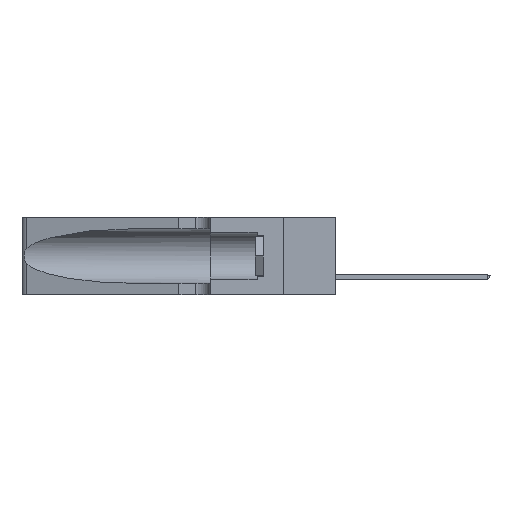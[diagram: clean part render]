
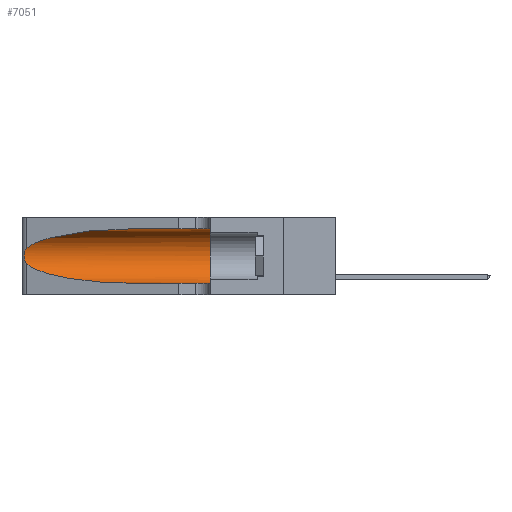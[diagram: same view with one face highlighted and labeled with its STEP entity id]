
A CAD part, left-side view. The second image highlights one B-rep face of the part: STEP entity #7051.
In plain terms, the highlighted cylindrical face has radius 3.308 mm (diameter 6.617 mm), a partial arc.
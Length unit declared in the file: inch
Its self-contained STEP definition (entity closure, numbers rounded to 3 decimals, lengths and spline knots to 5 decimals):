
#609 = CARTESIAN_POINT ( 'NONE',  ( 0.1305, 0.35, 0.31525 ) ) ;
#758 = CARTESIAN_POINT ( 'NONE',  ( 0.1305, 1.61858, 0.31525 ) ) ;
#1259 = AXIS2_PLACEMENT_3D ( 'NONE', #35674, #8339, #36142 ) ;
#1450 = CARTESIAN_POINT ( 'NONE',  ( 0.26075, 1.23896, 0.19203 ) ) ;
#2039 = CARTESIAN_POINT ( 'NONE',  ( 0.26075, 1.23896, 0.178 ) ) ;
#2385 = EDGE_CURVE ( 'NONE', #28341, #15840, #10176, .T. ) ;
#2926 = EDGE_CURVE ( 'NONE', #28791, #38067, #15833, .T. ) ;
#3540 = DIRECTION ( 'NONE',  ( 0., -1., 0. ) ) ;
#6143 = ORIENTED_EDGE ( 'NONE', *, *, #12284, .F. ) ;
#7031 = VERTEX_POINT ( 'NONE', #19176 ) ;
#7051 = ADVANCED_FACE ( 'NONE', ( #32981 ), #30847, .F. ) ;
#8081 = EDGE_CURVE ( 'NONE', #38067, #7031, #36028, .T. ) ;
#8339 = DIRECTION ( 'NONE',  ( 0., 1., 0. ) ) ;
#8526 = CARTESIAN_POINT ( 'NONE',  ( 0.26017, 1.23833, 0.17102 ) ) ;
#10176 = LINE ( 'NONE', #758, #22695 ) ;
#11030 = CARTESIAN_POINT ( 'NONE',  ( 0.1305, 0.72297, 0.31525 ) ) ;
#12284 = EDGE_CURVE ( 'NONE', #15840, #20941, #14368, .T. ) ;
#14368 = CIRCLE ( 'NONE', #1259, 0.13025 ) ;
#14975 = CARTESIAN_POINT ( 'NONE',  ( 0.25487, 1.22718, 0.22369 ) ) ;
#15460 = CARTESIAN_POINT ( 'NONE',  ( 0.25856, 1.23593, 0.16098 ) ) ;
#15833 = B_SPLINE_CURVE_WITH_KNOTS ( 'NONE', 3,
 ( #18590, #29553, #25940, #29239, #19055, #43270, #1450, #2039, #8526, #15460, #35856, #39640, #32686, #22611 ),
 .UNSPECIFIED., .F., .F.,
 ( 4, 2, 2, 2, 2, 2, 4 ),
 ( 0., 0.00027, 0.00053, 0.00107, 0.0016, 0.00187, 0.00214 ),
 .UNSPECIFIED. ) ;
#15840 = VERTEX_POINT ( 'NONE', #609 ) ;
#16563 = ORIENTED_EDGE ( 'NONE', *, *, #2926, .T. ) ;
#18590 = CARTESIAN_POINT ( 'NONE',  ( 0.25487, 1.22718, 0.22369 ) ) ;
#19055 = CARTESIAN_POINT ( 'NONE',  ( 0.25854, 1.2359, 0.20912 ) ) ;
#19176 = CARTESIAN_POINT ( 'NONE',  ( 0.1305, 0.72297, 0.05475 ) ) ;
#19561 = VECTOR ( 'NONE', #3540, 39.37008 ) ;
#20941 = VERTEX_POINT ( 'NONE', #39941 ) ;
#22208 = CARTESIAN_POINT ( 'NONE',  ( 0.1305, 0.72297, 0.05475 ) ) ;
#22611 = CARTESIAN_POINT ( 'NONE',  ( 0.25487, 1.22718, 0.14631 ) ) ;
#22695 = VECTOR ( 'NONE', #24949, 39.37008 ) ;
#24523 = AXIS2_PLACEMENT_3D ( 'NONE', #29678, #25906, #36593 ) ;
#24949 = DIRECTION ( 'NONE',  ( 0., -1., 0. ) ) ;
#25007 = CARTESIAN_POINT ( 'NONE',  ( 0.2373, 1.15595, 0.28018 ) ) ;
#25906 = DIRECTION ( 'NONE',  ( 0., -1., 0. ) ) ;
#25940 = CARTESIAN_POINT ( 'NONE',  ( 0.25639, 1.23184, 0.21858 ) ) ;
#26475 = ORIENTED_EDGE ( 'NONE', *, *, #43598, .T. ) ;
#28050 = EDGE_CURVE ( 'NONE', #28341, #28791, #36614, .T. ) ;
#28341 = VERTEX_POINT ( 'NONE', #39160 ) ;
#28791 = VERTEX_POINT ( 'NONE', #36741 ) ;
#29172 = CARTESIAN_POINT ( 'NONE',  ( 0.25487, 1.22718, 0.14631 ) ) ;
#29239 = CARTESIAN_POINT ( 'NONE',  ( 0.25787, 1.23484, 0.2124 ) ) ;
#29553 = CARTESIAN_POINT ( 'NONE',  ( 0.25555, 1.22994, 0.2215 ) ) ;
#29678 = CARTESIAN_POINT ( 'NONE',  ( 0.1305, 1.61858, 0.185 ) ) ;
#30847 = CYLINDRICAL_SURFACE ( 'NONE', #24523, 0.13025 ) ;
#31351 = CARTESIAN_POINT ( 'NONE',  ( 0.1305, 1.61858, 0.05475 ) ) ;
#32686 = CARTESIAN_POINT ( 'NONE',  ( 0.25555, 1.22993, 0.14849 ) ) ;
#32981 = FACE_OUTER_BOUND ( 'NONE', #39410, .T. ) ;
#34232 = ORIENTED_EDGE ( 'NONE', *, *, #2385, .F. ) ;
#34845 = ORIENTED_EDGE ( 'NONE', *, *, #28050, .T. ) ;
#35209 = CARTESIAN_POINT ( 'NONE',  ( 0.18966, 0.96281, 0.31525 ) ) ;
#35674 = CARTESIAN_POINT ( 'NONE',  ( 0.1305, 0.35, 0.185 ) ) ;
#35856 = CARTESIAN_POINT ( 'NONE',  ( 0.25789, 1.23486, 0.15765 ) ) ;
#36028 =( BOUNDED_CURVE ( )  B_SPLINE_CURVE ( 3, ( #29172, #42867, #36396, #22208 ),
 .UNSPECIFIED., .F., .T. ) 
 B_SPLINE_CURVE_WITH_KNOTS ( ( 4, 4 ),
 ( 3.44316, 4.71239 ),
 .UNSPECIFIED. ) 
 CURVE ( )  GEOMETRIC_REPRESENTATION_ITEM ( )  RATIONAL_B_SPLINE_CURVE ( ( 1., 0.87, 0.87, 1. ) ) 
 REPRESENTATION_ITEM ( '' )  );
#36142 = DIRECTION ( 'NONE',  ( 0., 0., 1. ) ) ;
#36396 = CARTESIAN_POINT ( 'NONE',  ( 0.18966, 0.96281, 0.05475 ) ) ;
#36593 = DIRECTION ( 'NONE',  ( 0., 0., -1. ) ) ;
#36614 =( BOUNDED_CURVE ( )  B_SPLINE_CURVE ( 3, ( #11030, #35209, #25007, #14975 ),
 .UNSPECIFIED., .F., .T. ) 
 B_SPLINE_CURVE_WITH_KNOTS ( ( 4, 4 ),
 ( 1.5708, 2.84003 ),
 .UNSPECIFIED. ) 
 CURVE ( )  GEOMETRIC_REPRESENTATION_ITEM ( )  RATIONAL_B_SPLINE_CURVE ( ( 1., 0.87, 0.87, 1. ) ) 
 REPRESENTATION_ITEM ( '' )  );
#36741 = CARTESIAN_POINT ( 'NONE',  ( 0.25487, 1.22718, 0.22369 ) ) ;
#37170 = CARTESIAN_POINT ( 'NONE',  ( 0.25487, 1.22718, 0.14631 ) ) ;
#38067 = VERTEX_POINT ( 'NONE', #37170 ) ;
#39160 = CARTESIAN_POINT ( 'NONE',  ( 0.1305, 0.72297, 0.31525 ) ) ;
#39410 = EDGE_LOOP ( 'NONE', ( #34845, #16563, #43724, #26475, #6143, #34232 ) ) ;
#39640 = CARTESIAN_POINT ( 'NONE',  ( 0.25639, 1.23186, 0.15144 ) ) ;
#39941 = CARTESIAN_POINT ( 'NONE',  ( 0.1305, 0.35, 0.05475 ) ) ;
#40148 = LINE ( 'NONE', #31351, #19561 ) ;
#42867 = CARTESIAN_POINT ( 'NONE',  ( 0.2373, 1.15595, 0.08982 ) ) ;
#43270 = CARTESIAN_POINT ( 'NONE',  ( 0.26018, 1.23835, 0.19895 ) ) ;
#43598 = EDGE_CURVE ( 'NONE', #7031, #20941, #40148, .T. ) ;
#43724 = ORIENTED_EDGE ( 'NONE', *, *, #8081, .T. ) ;
